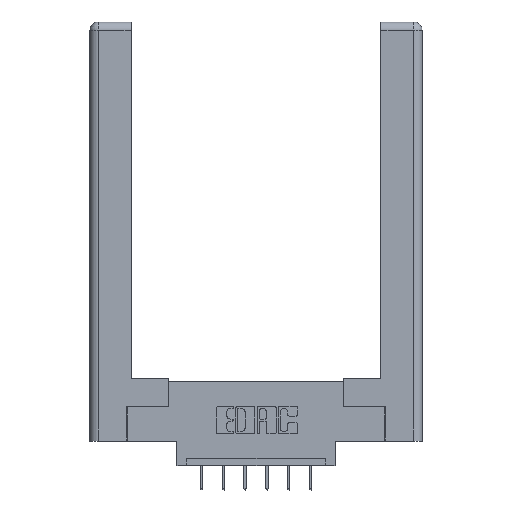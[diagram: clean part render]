
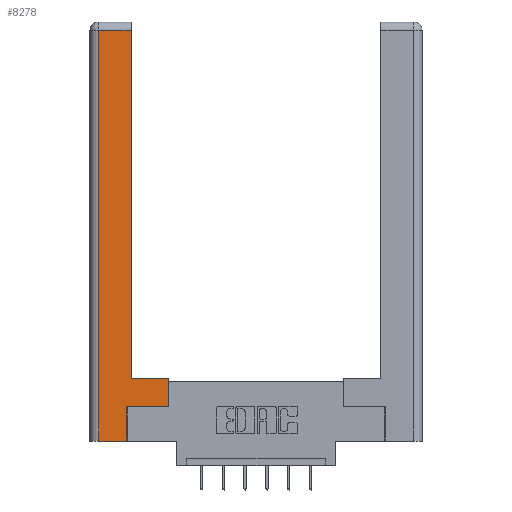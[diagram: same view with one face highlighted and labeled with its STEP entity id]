
A CAD part, top view. The second image highlights one B-rep face of the part: STEP entity #8278.
In plain terms, the highlighted planar face has unit normal (0, 0, 1).
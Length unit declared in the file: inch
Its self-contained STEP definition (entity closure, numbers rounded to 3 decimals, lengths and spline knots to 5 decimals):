
#115 = EDGE_LOOP ( 'NONE', ( #11915, #6790, #5102, #3310, #8260, #10153, #5697, #11124 ) ) ;
#377 = VERTEX_POINT ( 'NONE', #10024 ) ;
#437 = CARTESIAN_POINT ( 'NONE',  ( 0.295, 3., 0. ) ) ;
#453 = VECTOR ( 'NONE', #7724, 39.37008 ) ;
#460 = CARTESIAN_POINT ( 'NONE',  ( 0.565, 0.45, 0. ) ) ;
#526 = CARTESIAN_POINT ( 'NONE',  ( 0.265, 0., 0. ) ) ;
#614 = EDGE_CURVE ( 'NONE', #4595, #10418, #5382, .T. ) ;
#991 = DIRECTION ( 'NONE',  ( 0., -1., 0. ) ) ;
#1197 = LINE ( 'NONE', #3821, #2935 ) ;
#1613 = DIRECTION ( 'NONE',  ( -1., 0., 0. ) ) ;
#1808 = DIRECTION ( 'NONE',  ( 0., 1., 0. ) ) ;
#2069 = PLANE ( 'NONE',  #9088 ) ;
#2206 = LINE ( 'NONE', #5311, #9287 ) ;
#2285 = VECTOR ( 'NONE', #991, 39.37008 ) ;
#2300 = LINE ( 'NONE', #9624, #3174 ) ;
#2472 = CARTESIAN_POINT ( 'NONE',  ( 0.295, 0.45, 0. ) ) ;
#2935 = VECTOR ( 'NONE', #11239, 39.37008 ) ;
#3174 = VECTOR ( 'NONE', #7681, 39.37008 ) ;
#3310 = ORIENTED_EDGE ( 'NONE', *, *, #5412, .T. ) ;
#3423 = EDGE_CURVE ( 'NONE', #4762, #9655, #2206, .T. ) ;
#3702 = CARTESIAN_POINT ( 'NONE',  ( 0.0615, 0., 0. ) ) ;
#3723 = VERTEX_POINT ( 'NONE', #11830 ) ;
#3778 = EDGE_CURVE ( 'NONE', #377, #4762, #11297, .T. ) ;
#3821 = CARTESIAN_POINT ( 'NONE',  ( 0.0615, 2.94, 0. ) ) ;
#4269 = VECTOR ( 'NONE', #8854, 39.37008 ) ;
#4361 = EDGE_CURVE ( 'NONE', #3723, #6827, #1197, .T. ) ;
#4595 = VERTEX_POINT ( 'NONE', #526 ) ;
#4762 = VERTEX_POINT ( 'NONE', #460 ) ;
#5102 = ORIENTED_EDGE ( 'NONE', *, *, #7068, .T. ) ;
#5311 = CARTESIAN_POINT ( 'NONE',  ( 0.295, 0.45, 0. ) ) ;
#5382 = LINE ( 'NONE', #5927, #453 ) ;
#5412 = EDGE_CURVE ( 'NONE', #11455, #4595, #6672, .T. ) ;
#5697 = ORIENTED_EDGE ( 'NONE', *, *, #3778, .T. ) ;
#5806 = DIRECTION ( 'NONE',  ( 0., 0., -1. ) ) ;
#5927 = CARTESIAN_POINT ( 'NONE',  ( 0.265, 0.245, 0. ) ) ;
#6217 = FACE_OUTER_BOUND ( 'NONE', #115, .T. ) ;
#6672 = LINE ( 'NONE', #8734, #7092 ) ;
#6736 = DIRECTION ( 'NONE',  ( -1., 0., 0. ) ) ;
#6790 = ORIENTED_EDGE ( 'NONE', *, *, #4361, .T. ) ;
#6827 = VERTEX_POINT ( 'NONE', #8116 ) ;
#7068 = EDGE_CURVE ( 'NONE', #6827, #11455, #10928, .T. ) ;
#7092 = VECTOR ( 'NONE', #7781, 39.37008 ) ;
#7581 = CARTESIAN_POINT ( 'NONE',  ( 0., 0., 0. ) ) ;
#7681 = DIRECTION ( 'NONE',  ( 1., 0., 0. ) ) ;
#7701 = VECTOR ( 'NONE', #1808, 39.37008 ) ;
#7724 = DIRECTION ( 'NONE',  ( 0., 1., 0. ) ) ;
#7775 = EDGE_CURVE ( 'NONE', #10418, #377, #2300, .T. ) ;
#7781 = DIRECTION ( 'NONE',  ( 1., 0., 0. ) ) ;
#8116 = CARTESIAN_POINT ( 'NONE',  ( 0.0615, 2.94, 0. ) ) ;
#8260 = ORIENTED_EDGE ( 'NONE', *, *, #614, .T. ) ;
#8278 = ADVANCED_FACE ( 'NONE', ( #6217 ), #2069, .F. ) ;
#8734 = CARTESIAN_POINT ( 'NONE',  ( 0.265, 0., 0. ) ) ;
#8854 = DIRECTION ( 'NONE',  ( 0., 1., 0. ) ) ;
#8893 = LINE ( 'NONE', #437, #4269 ) ;
#9088 = AXIS2_PLACEMENT_3D ( 'NONE', #7581, #5806, #6736 ) ;
#9233 = CARTESIAN_POINT ( 'NONE',  ( 0.0615, 0., 0. ) ) ;
#9287 = VECTOR ( 'NONE', #1613, 39.37008 ) ;
#9624 = CARTESIAN_POINT ( 'NONE',  ( 0.565, 0.245, 0. ) ) ;
#9655 = VERTEX_POINT ( 'NONE', #2472 ) ;
#10024 = CARTESIAN_POINT ( 'NONE',  ( 0.565, 0.245, 0. ) ) ;
#10081 = EDGE_CURVE ( 'NONE', #9655, #3723, #8893, .T. ) ;
#10153 = ORIENTED_EDGE ( 'NONE', *, *, #7775, .T. ) ;
#10418 = VERTEX_POINT ( 'NONE', #11056 ) ;
#10928 = LINE ( 'NONE', #9233, #2285 ) ;
#11056 = CARTESIAN_POINT ( 'NONE',  ( 0.265, 0.245, 0. ) ) ;
#11124 = ORIENTED_EDGE ( 'NONE', *, *, #3423, .T. ) ;
#11169 = CARTESIAN_POINT ( 'NONE',  ( 0.565, 0.45, 0. ) ) ;
#11239 = DIRECTION ( 'NONE',  ( -1., 0., 0. ) ) ;
#11297 = LINE ( 'NONE', #11169, #7701 ) ;
#11455 = VERTEX_POINT ( 'NONE', #3702 ) ;
#11830 = CARTESIAN_POINT ( 'NONE',  ( 0.295, 2.94, 0. ) ) ;
#11915 = ORIENTED_EDGE ( 'NONE', *, *, #10081, .T. ) ;
